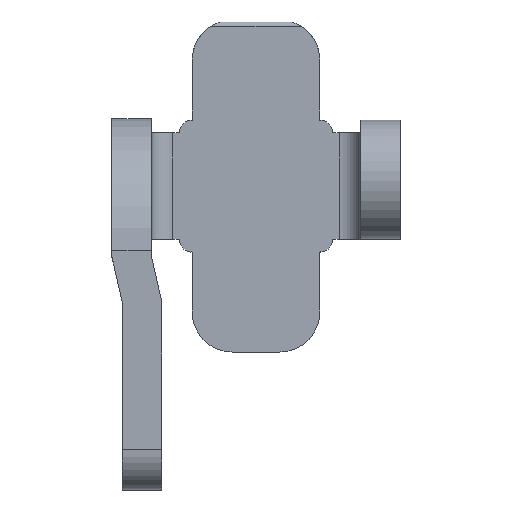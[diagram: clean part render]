
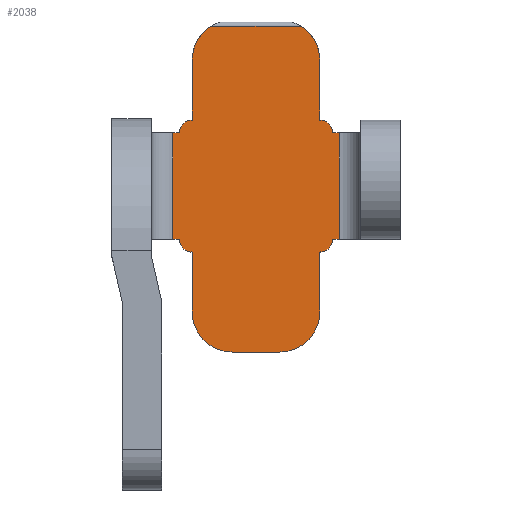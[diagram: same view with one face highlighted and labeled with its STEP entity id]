
A CAD part, top view. The second image highlights one B-rep face of the part: STEP entity #2038.
In plain terms, the highlighted planar face has unit normal (0, 0, 1).
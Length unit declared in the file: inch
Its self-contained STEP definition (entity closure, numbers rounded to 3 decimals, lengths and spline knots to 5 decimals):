
#643=CARTESIAN_POINT('',(0.206,0.686,0.093));
#644=DIRECTION('',(0.,0.,1.));
#645=DIRECTION('',(1.,0.,0.));
#646=AXIS2_PLACEMENT_3D('',#643,#644,#645);
#651=DIRECTION('',(0.,1.,0.));
#652=VECTOR('',#651,0.141);
#653=CARTESIAN_POINT('',(0.3,0.545,0.093));
#654=LINE('',#653,#652);
#658=CARTESIAN_POINT('',(0.3,0.515,0.093));
#659=DIRECTION('',(0.,0.,1.));
#660=DIRECTION('',(1.,0.,0.));
#661=AXIS2_PLACEMENT_3D('',#658,#659,#660);
#666=DIRECTION('',(-1.,0.,0.));
#667=VECTOR('',#666,0.016);
#668=CARTESIAN_POINT('',(0.346,0.515,0.093));
#669=LINE('',#668,#667);
#673=DIRECTION('',(1.,0.,0.));
#674=VECTOR('',#673,0.016);
#675=CARTESIAN_POINT('',(0.33,0.265,0.093));
#676=LINE('',#675,#674);
#680=CARTESIAN_POINT('',(0.3,0.265,0.093));
#681=DIRECTION('',(0.,0.,1.));
#682=DIRECTION('',(0.,-1.,0.));
#683=AXIS2_PLACEMENT_3D('',#680,#681,#682);
#688=DIRECTION('',(0.,1.,0.));
#689=VECTOR('',#688,0.141);
#690=CARTESIAN_POINT('',(0.3,0.094,0.093));
#691=LINE('',#690,#689);
#695=CARTESIAN_POINT('',(0.206,0.094,0.093));
#696=DIRECTION('',(0.,0.,1.));
#697=DIRECTION('',(0.,-1.,0.));
#698=AXIS2_PLACEMENT_3D('',#695,#696,#697);
#703=DIRECTION('',(1.,0.,0.));
#704=VECTOR('',#703,0.112);
#705=CARTESIAN_POINT('',(0.094,0.,0.093));
#706=LINE('',#705,#704);
#710=CARTESIAN_POINT('',(0.094,0.094,0.093));
#711=DIRECTION('',(0.,0.,1.));
#712=DIRECTION('',(-1.,0.,0.));
#713=AXIS2_PLACEMENT_3D('',#710,#711,#712);
#718=DIRECTION('',(0.,-1.,0.));
#719=VECTOR('',#718,0.141);
#720=CARTESIAN_POINT('',(0.,0.235,0.093));
#721=LINE('',#720,#719);
#725=CARTESIAN_POINT('',(0.,0.265,0.093));
#726=DIRECTION('',(0.,0.,1.));
#727=DIRECTION('',(-1.,0.,0.));
#728=AXIS2_PLACEMENT_3D('',#725,#726,#727);
#733=DIRECTION('',(1.,0.,0.));
#734=VECTOR('',#733,0.016);
#735=CARTESIAN_POINT('',(-0.046,0.265,0.093));
#736=LINE('',#735,#734);
#740=DIRECTION('',(-1.,0.,0.));
#741=VECTOR('',#740,0.016);
#742=CARTESIAN_POINT('',(-0.03,0.515,0.093));
#743=LINE('',#742,#741);
#747=CARTESIAN_POINT('',(0.,0.515,0.093));
#748=DIRECTION('',(0.,0.,1.));
#749=DIRECTION('',(0.,1.,0.));
#750=AXIS2_PLACEMENT_3D('',#747,#748,#749);
#755=DIRECTION('',(0.,-1.,0.));
#756=VECTOR('',#755,0.141);
#757=CARTESIAN_POINT('',(0.,0.686,0.093));
#758=LINE('',#757,#756);
#762=CARTESIAN_POINT('',(0.094,0.686,0.093));
#763=DIRECTION('',(0.,0.,1.));
#764=DIRECTION('',(-0.53,0.848,0.));
#765=AXIS2_PLACEMENT_3D('',#762,#763,#764);
#770=DIRECTION('',(1.,0.,0.));
#771=VECTOR('',#770,0.21162);
#772=CARTESIAN_POINT('',(0.04419,0.76572,0.093));
#773=LINE('',#772,#771);
#810=CARTESIAN_POINT('',(0.25581,0.76572,0.093));
#842=CARTESIAN_POINT('',(0.04419,0.76572,0.093));
#1088=DIRECTION('',(0.,-1.,0.));
#1089=VECTOR('',#1088,0.25);
#1090=CARTESIAN_POINT('',(0.346,0.515,0.093));
#1091=LINE('',#1090,#1089);
#1307=DIRECTION('',(0.,1.,0.));
#1308=VECTOR('',#1307,0.25);
#1309=CARTESIAN_POINT('',(-0.046,0.265,0.093));
#1310=LINE('',#1309,#1308);
#1410=CARTESIAN_POINT('',(0.,0.094,0.093));
#1411=VERTEX_POINT('',#1410);
#1412=CARTESIAN_POINT('',(0.,0.235,0.093));
#1413=VERTEX_POINT('',#1412);
#1414=CARTESIAN_POINT('',(0.094,0.,0.093));
#1415=VERTEX_POINT('',#1414);
#1416=CARTESIAN_POINT('',(0.206,0.,0.093));
#1417=VERTEX_POINT('',#1416);
#1418=CARTESIAN_POINT('',(0.3,0.094,0.093));
#1419=VERTEX_POINT('',#1418);
#1420=CARTESIAN_POINT('',(0.3,0.235,0.093));
#1421=VERTEX_POINT('',#1420);
#1423=VERTEX_POINT('',#810);
#1428=VERTEX_POINT('',#842);
#1432=CARTESIAN_POINT('',(0.,0.686,0.093));
#1433=VERTEX_POINT('',#1432);
#1439=CARTESIAN_POINT('',(-0.046,0.515,0.093));
#1440=VERTEX_POINT('',#1439);
#1441=CARTESIAN_POINT('',(-0.03,0.515,0.093));
#1442=VERTEX_POINT('',#1441);
#1455=CARTESIAN_POINT('',(-0.03,0.265,0.093));
#1456=VERTEX_POINT('',#1455);
#1457=CARTESIAN_POINT('',(-0.046,0.265,0.093));
#1458=VERTEX_POINT('',#1457);
#1465=CARTESIAN_POINT('',(0.346,0.265,0.093));
#1466=VERTEX_POINT('',#1465);
#1467=CARTESIAN_POINT('',(0.33,0.265,0.093));
#1468=VERTEX_POINT('',#1467);
#1491=CARTESIAN_POINT('',(0.33,0.515,0.093));
#1492=VERTEX_POINT('',#1491);
#1493=CARTESIAN_POINT('',(0.346,0.515,0.093));
#1494=VERTEX_POINT('',#1493);
#1503=CARTESIAN_POINT('',(0.,0.545,0.093));
#1504=VERTEX_POINT('',#1503);
#1505=CARTESIAN_POINT('',(0.3,0.545,0.093));
#1506=VERTEX_POINT('',#1505);
#1507=CARTESIAN_POINT('',(0.3,0.686,0.093));
#1508=VERTEX_POINT('',#1507);
#1994=CARTESIAN_POINT('',(0.346,0.515,0.093));
#1995=DIRECTION('',(0.,0.,-1.));
#1996=DIRECTION('',(-1.,0.,0.));
#1997=AXIS2_PLACEMENT_3D('',#1994,#1995,#1996);
#1998=PLANE('',#1997);
#2000=ORIENTED_EDGE('',*,*,#1999,.T.);
#2002=ORIENTED_EDGE('',*,*,#2001,.F.);
#2004=ORIENTED_EDGE('',*,*,#2003,.F.);
#2006=ORIENTED_EDGE('',*,*,#2005,.F.);
#2008=ORIENTED_EDGE('',*,*,#2007,.F.);
#2010=ORIENTED_EDGE('',*,*,#2009,.T.);
#2012=ORIENTED_EDGE('',*,*,#2011,.F.);
#2014=ORIENTED_EDGE('',*,*,#2013,.F.);
#2016=ORIENTED_EDGE('',*,*,#2015,.F.);
#2018=ORIENTED_EDGE('',*,*,#2017,.F.);
#2020=ORIENTED_EDGE('',*,*,#2019,.F.);
#2022=ORIENTED_EDGE('',*,*,#2021,.F.);
#2024=ORIENTED_EDGE('',*,*,#2023,.F.);
#2025=ORIENTED_EDGE('',*,*,#1981,.F.);
#2026=ORIENTED_EDGE('',*,*,#1789,.F.);
#2028=ORIENTED_EDGE('',*,*,#2027,.T.);
#2029=ORIENTED_EDGE('',*,*,#1827,.F.);
#2031=ORIENTED_EDGE('',*,*,#2030,.F.);
#2033=ORIENTED_EDGE('',*,*,#2032,.F.);
#2035=ORIENTED_EDGE('',*,*,#2034,.F.);
#2036=EDGE_LOOP('',(#2000,#2002,#2004,#2006,#2008,#2010,#2012,#2014,#2016,#2018,
#2020,#2022,#2024,#2025,#2026,#2028,#2029,#2031,#2033,#2035));
#2037=FACE_OUTER_BOUND('',#2036,.F.);
#647=CIRCLE('',#646,0.094);
#662=CIRCLE('',#661,0.03);
#684=CIRCLE('',#683,0.03);
#699=CIRCLE('',#698,0.094);
#714=CIRCLE('',#713,0.094);
#729=CIRCLE('',#728,0.03);
#751=CIRCLE('',#750,0.03);
#766=CIRCLE('',#765,0.094);
#1789=EDGE_CURVE('',#1458,#1456,#736,.T.);
#1827=EDGE_CURVE('',#1442,#1440,#743,.T.);
#1981=EDGE_CURVE('',#1456,#1413,#729,.T.);
#1999=EDGE_CURVE('',#1428,#1423,#773,.T.);
#2001=EDGE_CURVE('',#1508,#1423,#647,.T.);
#2003=EDGE_CURVE('',#1506,#1508,#654,.T.);
#2005=EDGE_CURVE('',#1492,#1506,#662,.T.);
#2007=EDGE_CURVE('',#1494,#1492,#669,.T.);
#2009=EDGE_CURVE('',#1494,#1466,#1091,.T.);
#2011=EDGE_CURVE('',#1468,#1466,#676,.T.);
#2013=EDGE_CURVE('',#1421,#1468,#684,.T.);
#2015=EDGE_CURVE('',#1419,#1421,#691,.T.);
#2017=EDGE_CURVE('',#1417,#1419,#699,.T.);
#2019=EDGE_CURVE('',#1415,#1417,#706,.T.);
#2021=EDGE_CURVE('',#1411,#1415,#714,.T.);
#2023=EDGE_CURVE('',#1413,#1411,#721,.T.);
#2027=EDGE_CURVE('',#1458,#1440,#1310,.T.);
#2030=EDGE_CURVE('',#1504,#1442,#751,.T.);
#2032=EDGE_CURVE('',#1433,#1504,#758,.T.);
#2034=EDGE_CURVE('',#1428,#1433,#766,.T.);
#2038=ADVANCED_FACE('',(#2037),#1998,.F.);
